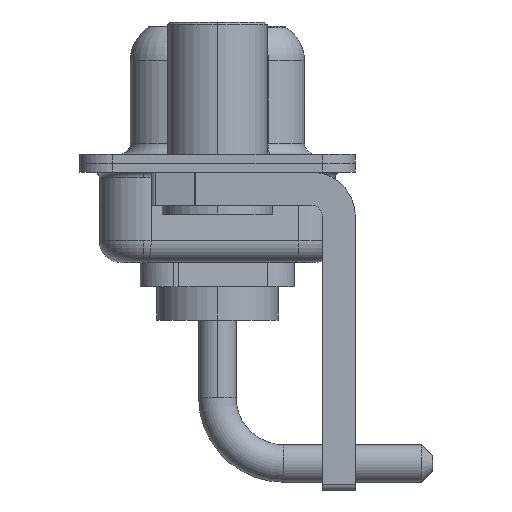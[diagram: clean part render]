
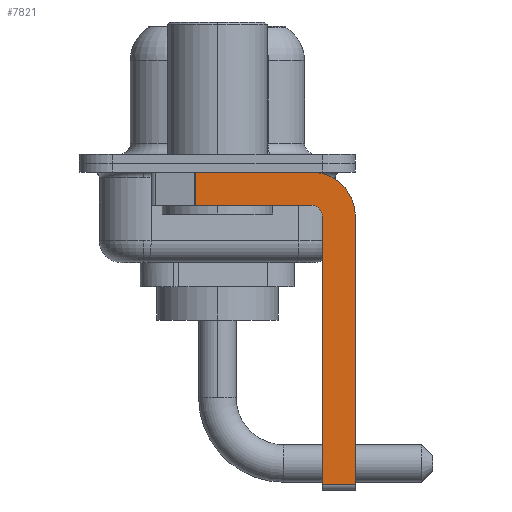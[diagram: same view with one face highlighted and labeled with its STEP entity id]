
A CAD part, left-side view. The second image highlights one B-rep face of the part: STEP entity #7821.
In plain terms, the highlighted planar face has unit normal (-1, 0, 0).
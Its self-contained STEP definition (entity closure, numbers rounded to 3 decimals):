
#11 = DIRECTION ( 'NONE',  ( 0., 0., -1. ) ) ;
#344 = EDGE_CURVE ( 'NONE', #638, #8098, #4732, .T. ) ;
#638 = VERTEX_POINT ( 'NONE', #8310 ) ;
#748 = LINE ( 'NONE', #5332, #11733 ) ;
#1168 = ORIENTED_EDGE ( 'NONE', *, *, #5182, .F. ) ;
#1236 = FACE_OUTER_BOUND ( 'NONE', #3306, .T. ) ;
#1387 = VERTEX_POINT ( 'NONE', #12741 ) ;
#1755 = CARTESIAN_POINT ( 'NONE',  ( -2.9, -4.25, -2.4 ) ) ;
#2424 = CARTESIAN_POINT ( 'NONE',  ( -2.9, -4.25, -2.4 ) ) ;
#2806 = CARTESIAN_POINT ( 'NONE',  ( -2.9, 3., -0.4 ) ) ;
#2957 = DIRECTION ( 'NONE',  ( 0., -1., 0. ) ) ;
#3080 = VECTOR ( 'NONE', #14792, 1000. ) ;
#3246 = VECTOR ( 'NONE', #7628, 1000. ) ;
#3268 = CARTESIAN_POINT ( 'NONE',  ( -2.9, -4.25, -0.4 ) ) ;
#3306 = EDGE_LOOP ( 'NONE', ( #14637, #9233, #4224, #6783, #10416, #8266, #1168, #14233 ) ) ;
#3330 = EDGE_CURVE ( 'NONE', #14054, #8098, #4376, .T. ) ;
#3618 = VERTEX_POINT ( 'NONE', #12088 ) ;
#3887 = AXIS2_PLACEMENT_3D ( 'NONE', #2424, #5815, #7087 ) ;
#4224 = ORIENTED_EDGE ( 'NONE', *, *, #3330, .F. ) ;
#4351 = CARTESIAN_POINT ( 'NONE',  ( -2.9, -4.75, -2.4 ) ) ;
#4376 = LINE ( 'NONE', #12575, #3080 ) ;
#4732 = LINE ( 'NONE', #11561, #8202 ) ;
#4902 = EDGE_CURVE ( 'NONE', #5365, #11459, #748, .T. ) ;
#5182 = EDGE_CURVE ( 'NONE', #1387, #3618, #5557, .T. ) ;
#5332 = CARTESIAN_POINT ( 'NONE',  ( -2.9, -4.75, -14.8 ) ) ;
#5359 = AXIS2_PLACEMENT_3D ( 'NONE', #1755, #7603, #9781 ) ;
#5365 = VERTEX_POINT ( 'NONE', #10434 ) ;
#5456 = CARTESIAN_POINT ( 'NONE',  ( -2.9, -4.25, -14.55 ) ) ;
#5557 = LINE ( 'NONE', #8014, #6459 ) ;
#5815 = DIRECTION ( 'NONE',  ( 1., 0., 0. ) ) ;
#6459 = VECTOR ( 'NONE', #11, 1000. ) ;
#6783 = ORIENTED_EDGE ( 'NONE', *, *, #10816, .F. ) ;
#7087 = DIRECTION ( 'NONE',  ( 0., 0., -1. ) ) ;
#7525 = AXIS2_PLACEMENT_3D ( 'NONE', #13619, #8223, #12396 ) ;
#7553 = EDGE_CURVE ( 'NONE', #638, #14117, #13135, .T. ) ;
#7603 = DIRECTION ( 'NONE',  ( -1., 0., 0. ) ) ;
#7628 = DIRECTION ( 'NONE',  ( 0., -1., 0. ) ) ;
#7821 = ADVANCED_FACE ( 'NONE', ( #1236 ), #8199, .F. ) ;
#7878 = DIRECTION ( 'NONE',  ( 0., 0., -1. ) ) ;
#7996 = CIRCLE ( 'NONE', #7525, 2. ) ;
#8014 = CARTESIAN_POINT ( 'NONE',  ( -2.9, -6.25, -2.4 ) ) ;
#8098 = VERTEX_POINT ( 'NONE', #8994 ) ;
#8199 = PLANE ( 'NONE',  #3887 ) ;
#8202 = VECTOR ( 'NONE', #7878, 1000. ) ;
#8223 = DIRECTION ( 'NONE',  ( 1., 0., 0. ) ) ;
#8266 = ORIENTED_EDGE ( 'NONE', *, *, #14400, .T. ) ;
#8310 = CARTESIAN_POINT ( 'NONE',  ( -2.9, 0.978, -0.4 ) ) ;
#8994 = CARTESIAN_POINT ( 'NONE',  ( -2.9, 0.978, -1.9 ) ) ;
#9233 = ORIENTED_EDGE ( 'NONE', *, *, #344, .T. ) ;
#9781 = DIRECTION ( 'NONE',  ( 0., 0., 1. ) ) ;
#10148 = EDGE_CURVE ( 'NONE', #14117, #1387, #7996, .T. ) ;
#10416 = ORIENTED_EDGE ( 'NONE', *, *, #4902, .F. ) ;
#10434 = CARTESIAN_POINT ( 'NONE',  ( -2.9, -4.75, -14.55 ) ) ;
#10648 = LINE ( 'NONE', #5456, #3246 ) ;
#10816 = EDGE_CURVE ( 'NONE', #11459, #14054, #13780, .T. ) ;
#11321 = CARTESIAN_POINT ( 'NONE',  ( -2.9, -4.25, -1.9 ) ) ;
#11459 = VERTEX_POINT ( 'NONE', #4351 ) ;
#11561 = CARTESIAN_POINT ( 'NONE',  ( -2.9, 0.978, -1.9 ) ) ;
#11733 = VECTOR ( 'NONE', #13610, 1000. ) ;
#12088 = CARTESIAN_POINT ( 'NONE',  ( -2.9, -6.25, -14.55 ) ) ;
#12396 = DIRECTION ( 'NONE',  ( 0., 0., -1. ) ) ;
#12575 = CARTESIAN_POINT ( 'NONE',  ( -2.9, -4.25, -1.9 ) ) ;
#12741 = CARTESIAN_POINT ( 'NONE',  ( -2.9, -6.25, -2.4 ) ) ;
#13014 = VECTOR ( 'NONE', #2957, 1000. ) ;
#13135 = LINE ( 'NONE', #2806, #13014 ) ;
#13610 = DIRECTION ( 'NONE',  ( 0., 0., 1. ) ) ;
#13619 = CARTESIAN_POINT ( 'NONE',  ( -2.9, -4.25, -2.4 ) ) ;
#13780 = CIRCLE ( 'NONE', #5359, 0.5 ) ;
#14054 = VERTEX_POINT ( 'NONE', #11321 ) ;
#14117 = VERTEX_POINT ( 'NONE', #3268 ) ;
#14233 = ORIENTED_EDGE ( 'NONE', *, *, #10148, .F. ) ;
#14400 = EDGE_CURVE ( 'NONE', #5365, #3618, #10648, .T. ) ;
#14637 = ORIENTED_EDGE ( 'NONE', *, *, #7553, .F. ) ;
#14792 = DIRECTION ( 'NONE',  ( 0., 1., 0. ) ) ;
